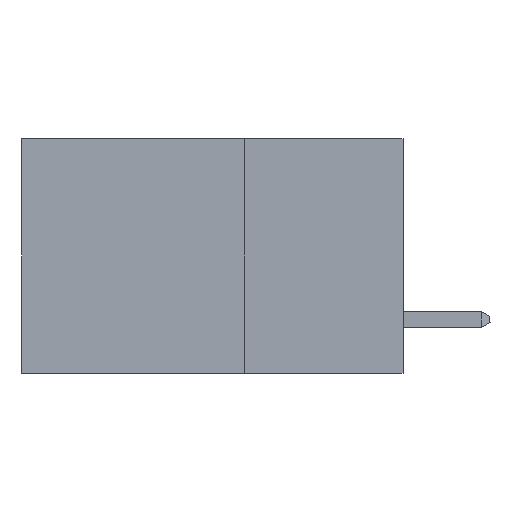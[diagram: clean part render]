
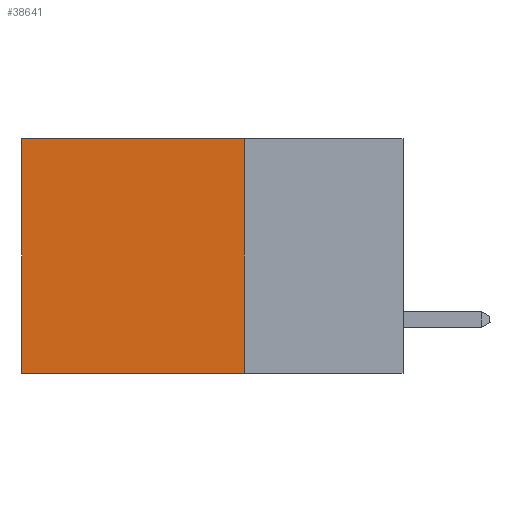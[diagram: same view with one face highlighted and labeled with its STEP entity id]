
A CAD part, left-side view. The second image highlights one B-rep face of the part: STEP entity #38641.
In plain terms, the highlighted planar face has unit normal (-1, 0, 0).
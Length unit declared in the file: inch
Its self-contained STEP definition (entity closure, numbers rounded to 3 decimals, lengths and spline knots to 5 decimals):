
#542 = CARTESIAN_POINT ( 'NONE',  ( 0.2875, 0.25, 0. ) ) ;
#1989 = FACE_OUTER_BOUND ( 'NONE', #19783, .T. ) ;
#4024 = DIRECTION ( 'NONE',  ( 1., 0., 0. ) ) ;
#4561 = VERTEX_POINT ( 'NONE', #542 ) ;
#7623 = VECTOR ( 'NONE', #11910, 39.37008 ) ;
#7873 = CARTESIAN_POINT ( 'NONE',  ( 0.2875, 0.6, 0. ) ) ;
#8760 = LINE ( 'NONE', #7873, #37335 ) ;
#10273 = VECTOR ( 'NONE', #43995, 39.37008 ) ;
#11054 = PLANE ( 'NONE',  #21325 ) ;
#11910 = DIRECTION ( 'NONE',  ( 0., 0., -1. ) ) ;
#12038 = LINE ( 'NONE', #23406, #31916 ) ;
#12215 = ORIENTED_EDGE ( 'NONE', *, *, #36619, .T. ) ;
#12759 = EDGE_CURVE ( 'NONE', #35690, #22921, #8760, .T. ) ;
#13091 = CARTESIAN_POINT ( 'NONE',  ( 0.2875, 0.25, -0.37 ) ) ;
#16987 = VERTEX_POINT ( 'NONE', #13091 ) ;
#17212 = ORIENTED_EDGE ( 'NONE', *, *, #34355, .F. ) ;
#19783 = EDGE_LOOP ( 'NONE', ( #21385, #35681, #17212, #12215 ) ) ;
#20305 = DIRECTION ( 'NONE',  ( 0., 1., 0. ) ) ;
#21325 = AXIS2_PLACEMENT_3D ( 'NONE', #40892, #4024, #41375 ) ;
#21385 = ORIENTED_EDGE ( 'NONE', *, *, #12759, .T. ) ;
#21513 = CARTESIAN_POINT ( 'NONE',  ( 0.2875, 0.25, 0. ) ) ;
#22087 = DIRECTION ( 'NONE',  ( 0., 0., -1. ) ) ;
#22921 = VERTEX_POINT ( 'NONE', #25963 ) ;
#23406 = CARTESIAN_POINT ( 'NONE',  ( 0.2875, 0.25, -0.37 ) ) ;
#25963 = CARTESIAN_POINT ( 'NONE',  ( 0.2875, 0.6, -0.37 ) ) ;
#28992 = LINE ( 'NONE', #21513, #10273 ) ;
#31916 = VECTOR ( 'NONE', #20305, 39.37008 ) ;
#34355 = EDGE_CURVE ( 'NONE', #4561, #16987, #40378, .T. ) ;
#35681 = ORIENTED_EDGE ( 'NONE', *, *, #36981, .F. ) ;
#35690 = VERTEX_POINT ( 'NONE', #46285 ) ;
#36619 = EDGE_CURVE ( 'NONE', #4561, #35690, #28992, .T. ) ;
#36981 = EDGE_CURVE ( 'NONE', #16987, #22921, #12038, .T. ) ;
#37335 = VECTOR ( 'NONE', #22087, 39.37008 ) ;
#38641 = ADVANCED_FACE ( 'NONE', ( #1989 ), #11054, .F. ) ;
#40378 = LINE ( 'NONE', #44580, #7623 ) ;
#40892 = CARTESIAN_POINT ( 'NONE',  ( 0.2875, 0.25, 0. ) ) ;
#41375 = DIRECTION ( 'NONE',  ( 0., 0., -1. ) ) ;
#43995 = DIRECTION ( 'NONE',  ( 0., 1., 0. ) ) ;
#44580 = CARTESIAN_POINT ( 'NONE',  ( 0.2875, 0.25, 0. ) ) ;
#46285 = CARTESIAN_POINT ( 'NONE',  ( 0.2875, 0.6, 0. ) ) ;
